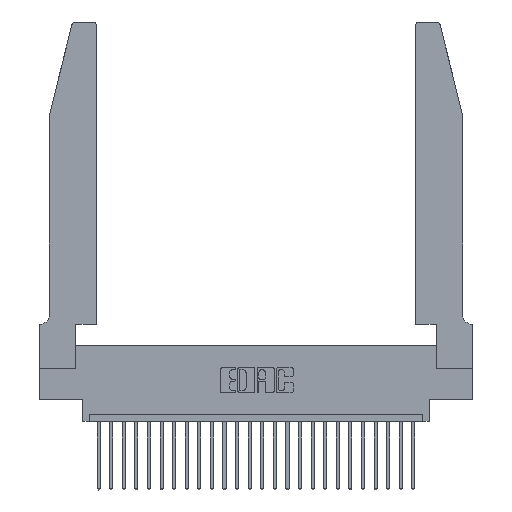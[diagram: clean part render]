
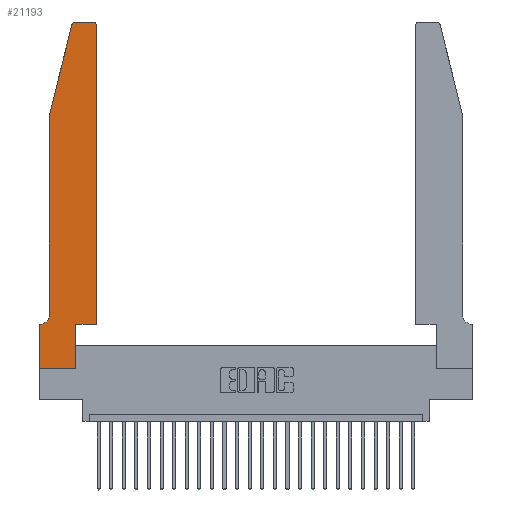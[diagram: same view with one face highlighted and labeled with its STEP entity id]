
A CAD part, top view. The second image highlights one B-rep face of the part: STEP entity #21193.
In plain terms, the highlighted planar face has unit normal (0, 0, 1).
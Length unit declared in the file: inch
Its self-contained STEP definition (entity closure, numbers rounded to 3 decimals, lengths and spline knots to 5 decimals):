
#7 = VECTOR ( 'NONE', #18177, 39.37008 ) ;
#170 = CARTESIAN_POINT ( 'NONE',  ( 0.0755, 0.35, 0.37 ) ) ;
#530 = ORIENTED_EDGE ( 'NONE', *, *, #626, .T. ) ;
#626 = EDGE_CURVE ( 'NONE', #14265, #8389, #19176, .T. ) ;
#1041 = CARTESIAN_POINT ( 'NONE',  ( 0.4505, 0.35, 0.37 ) ) ;
#1094 = VERTEX_POINT ( 'NONE', #22489 ) ;
#1299 = DIRECTION ( 'NONE',  ( 1., 0., 0. ) ) ;
#1550 = DIRECTION ( 'NONE',  ( 0., 0., 1. ) ) ;
#1741 = DIRECTION ( 'NONE',  ( -1., 0., 0. ) ) ;
#1790 = CARTESIAN_POINT ( 'NONE',  ( 0.0755, 0.42, 0.37 ) ) ;
#2440 = DIRECTION ( 'NONE',  ( 0., -1., 0. ) ) ;
#2649 = DIRECTION ( 'NONE',  ( 0., 0., 1. ) ) ;
#2818 = ORIENTED_EDGE ( 'NONE', *, *, #4582, .T. ) ;
#3182 = CARTESIAN_POINT ( 'NONE',  ( 0.0055, 0.35, 0.37 ) ) ;
#3458 = PLANE ( 'NONE',  #10916 ) ;
#3552 = CARTESIAN_POINT ( 'NONE',  ( 0.4205, 2.72, 0.37 ) ) ;
#3847 = ORIENTED_EDGE ( 'NONE', *, *, #6996, .T. ) ;
#4052 = EDGE_CURVE ( 'NONE', #15006, #21285, #11974, .T. ) ;
#4496 = LINE ( 'NONE', #18867, #19284 ) ;
#4582 = EDGE_CURVE ( 'NONE', #5017, #15006, #19060, .T. ) ;
#5017 = VERTEX_POINT ( 'NONE', #10710 ) ;
#5562 = DIRECTION ( 'NONE',  ( 1., 0., 0. ) ) ;
#5655 = DIRECTION ( 'NONE',  ( 0., 0., -1. ) ) ;
#6118 = CARTESIAN_POINT ( 'NONE',  ( 0.4505, 0.35, 0.37 ) ) ;
#6258 = CARTESIAN_POINT ( 'NONE',  ( 0., 0., 0.37 ) ) ;
#6996 = EDGE_CURVE ( 'NONE', #21285, #12282, #8922, .T. ) ;
#7100 = VERTEX_POINT ( 'NONE', #14620 ) ;
#7427 = LINE ( 'NONE', #6258, #23190 ) ;
#7545 = AXIS2_PLACEMENT_3D ( 'NONE', #17927, #5655, #1741 ) ;
#7607 = ORIENTED_EDGE ( 'NONE', *, *, #17349, .T. ) ;
#8389 = VERTEX_POINT ( 'NONE', #1041 ) ;
#8882 = ORIENTED_EDGE ( 'NONE', *, *, #12635, .T. ) ;
#8922 = LINE ( 'NONE', #170, #21182 ) ;
#8928 = LINE ( 'NONE', #6118, #13093 ) ;
#9010 = VERTEX_POINT ( 'NONE', #18634 ) ;
#9364 = CARTESIAN_POINT ( 'NONE',  ( 0., 0.35, 0.37 ) ) ;
#9528 = CARTESIAN_POINT ( 'NONE',  ( 0., 0., 0.37 ) ) ;
#9646 = LINE ( 'NONE', #24203, #7 ) ;
#9731 = EDGE_LOOP ( 'NONE', ( #7607, #19654, #8882, #2818, #25338, #3847, #23391, #20321, #15099, #530, #10422, #24447 ) ) ;
#10140 = CARTESIAN_POINT ( 'NONE',  ( 0.2865, 0.35, 0.37 ) ) ;
#10180 = CIRCLE ( 'NONE', #19137, 0.03 ) ;
#10400 = DIRECTION ( 'NONE',  ( -1., 0., 0. ) ) ;
#10422 = ORIENTED_EDGE ( 'NONE', *, *, #24472, .T. ) ;
#10612 = DIRECTION ( 'NONE',  ( 1., 0., 0. ) ) ;
#10710 = CARTESIAN_POINT ( 'NONE',  ( 0.0755, 2., 0.37 ) ) ;
#10799 = CARTESIAN_POINT ( 'NONE',  ( 0.284, 2.72, 0.37 ) ) ;
#10916 = AXIS2_PLACEMENT_3D ( 'NONE', #9364, #11683, #1299 ) ;
#11444 = VECTOR ( 'NONE', #18294, 39.37008 ) ;
#11481 = VERTEX_POINT ( 'NONE', #9528 ) ;
#11683 = DIRECTION ( 'NONE',  ( 0., 0., 1. ) ) ;
#11974 = CIRCLE ( 'NONE', #7545, 0.07 ) ;
#12282 = VERTEX_POINT ( 'NONE', #15014 ) ;
#12635 = EDGE_CURVE ( 'NONE', #1094, #5017, #4496, .T. ) ;
#13093 = VECTOR ( 'NONE', #26397, 39.37008 ) ;
#14233 = CARTESIAN_POINT ( 'NONE',  ( 0.2865, 0.35, 0.37 ) ) ;
#14265 = VERTEX_POINT ( 'NONE', #10140 ) ;
#14471 = CARTESIAN_POINT ( 'NONE',  ( 0., 0., 0.37 ) ) ;
#14620 = CARTESIAN_POINT ( 'NONE',  ( 0.4205, 2.75, 0.37 ) ) ;
#14669 = LINE ( 'NONE', #14471, #22098 ) ;
#15006 = VERTEX_POINT ( 'NONE', #1790 ) ;
#15014 = CARTESIAN_POINT ( 'NONE',  ( 0., 0.35, 0.37 ) ) ;
#15099 = ORIENTED_EDGE ( 'NONE', *, *, #20006, .T. ) ;
#15882 = CARTESIAN_POINT ( 'NONE',  ( 0.284, 2.75, 0.37 ) ) ;
#16125 = CIRCLE ( 'NONE', #22896, 0.03 ) ;
#16190 = EDGE_CURVE ( 'NONE', #25524, #1094, #16125, .T. ) ;
#16936 = LINE ( 'NONE', #14233, #11444 ) ;
#16971 = DIRECTION ( 'NONE',  ( -0.239, -0.971, 0. ) ) ;
#17032 = DIRECTION ( 'NONE',  ( 1., 0., 0. ) ) ;
#17184 = CARTESIAN_POINT ( 'NONE',  ( 0.4505, 0.35, 0.37 ) ) ;
#17349 = EDGE_CURVE ( 'NONE', #7100, #25524, #9646, .T. ) ;
#17702 = CARTESIAN_POINT ( 'NONE',  ( 0.4505, 2.72, 0.37 ) ) ;
#17754 = VECTOR ( 'NONE', #17889, 39.37008 ) ;
#17889 = DIRECTION ( 'NONE',  ( 0., -1., 0. ) ) ;
#17927 = CARTESIAN_POINT ( 'NONE',  ( 0.0055, 0.42, 0.37 ) ) ;
#18177 = DIRECTION ( 'NONE',  ( -1., 0., 0. ) ) ;
#18294 = DIRECTION ( 'NONE',  ( 0., 1., 0. ) ) ;
#18634 = CARTESIAN_POINT ( 'NONE',  ( 0.2865, 0., 0.37 ) ) ;
#18705 = VERTEX_POINT ( 'NONE', #17702 ) ;
#18867 = CARTESIAN_POINT ( 'NONE',  ( 0.0755, 2., 0.37 ) ) ;
#19060 = LINE ( 'NONE', #21860, #17754 ) ;
#19137 = AXIS2_PLACEMENT_3D ( 'NONE', #3552, #1550, #5562 ) ;
#19176 = LINE ( 'NONE', #17184, #24312 ) ;
#19284 = VECTOR ( 'NONE', #16971, 39.37008 ) ;
#19654 = ORIENTED_EDGE ( 'NONE', *, *, #16190, .T. ) ;
#20006 = EDGE_CURVE ( 'NONE', #9010, #14265, #16936, .T. ) ;
#20321 = ORIENTED_EDGE ( 'NONE', *, *, #23244, .T. ) ;
#21182 = VECTOR ( 'NONE', #10400, 39.37008 ) ;
#21193 = ADVANCED_FACE ( 'NONE', ( #23600 ), #3458, .T. ) ;
#21285 = VERTEX_POINT ( 'NONE', #3182 ) ;
#21860 = CARTESIAN_POINT ( 'NONE',  ( 0.0755, 2., 0.37 ) ) ;
#22098 = VECTOR ( 'NONE', #2440, 39.37008 ) ;
#22489 = CARTESIAN_POINT ( 'NONE',  ( 0.25487, 2.72718, 0.37 ) ) ;
#22896 = AXIS2_PLACEMENT_3D ( 'NONE', #10799, #2649, #17032 ) ;
#23190 = VECTOR ( 'NONE', #10612, 39.37008 ) ;
#23244 = EDGE_CURVE ( 'NONE', #11481, #9010, #7427, .T. ) ;
#23376 = DIRECTION ( 'NONE',  ( 1., 0., 0. ) ) ;
#23391 = ORIENTED_EDGE ( 'NONE', *, *, #25184, .T. ) ;
#23600 = FACE_OUTER_BOUND ( 'NONE', #9731, .T. ) ;
#24203 = CARTESIAN_POINT ( 'NONE',  ( 0.2605, 2.75, 0.37 ) ) ;
#24312 = VECTOR ( 'NONE', #23376, 39.37008 ) ;
#24447 = ORIENTED_EDGE ( 'NONE', *, *, #24915, .T. ) ;
#24472 = EDGE_CURVE ( 'NONE', #8389, #18705, #8928, .T. ) ;
#24915 = EDGE_CURVE ( 'NONE', #18705, #7100, #10180, .T. ) ;
#25184 = EDGE_CURVE ( 'NONE', #12282, #11481, #14669, .T. ) ;
#25338 = ORIENTED_EDGE ( 'NONE', *, *, #4052, .T. ) ;
#25524 = VERTEX_POINT ( 'NONE', #15882 ) ;
#26397 = DIRECTION ( 'NONE',  ( 0., 1., 0. ) ) ;
